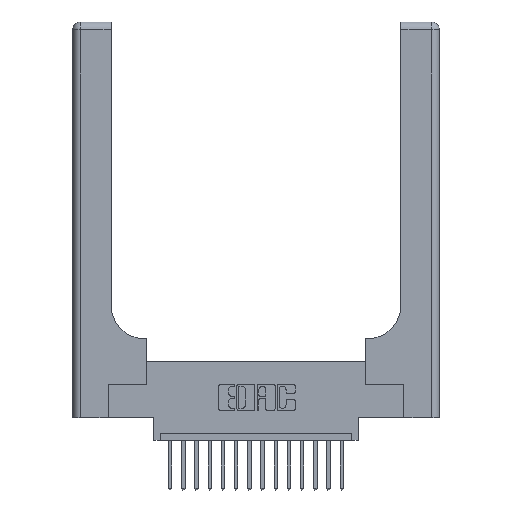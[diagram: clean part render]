
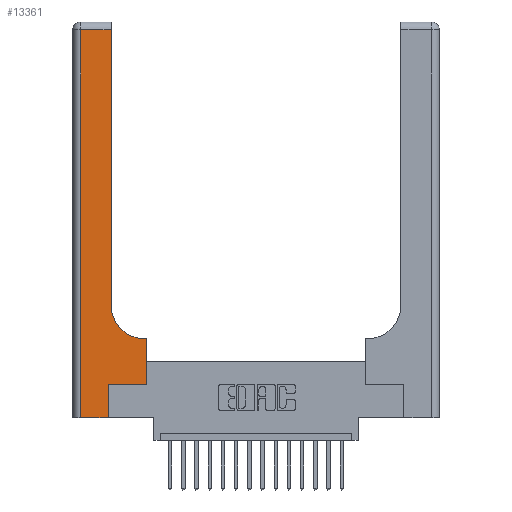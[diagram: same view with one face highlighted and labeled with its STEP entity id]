
A CAD part, top view. The second image highlights one B-rep face of the part: STEP entity #13361.
In plain terms, the highlighted planar face has unit normal (0, 0, 1).
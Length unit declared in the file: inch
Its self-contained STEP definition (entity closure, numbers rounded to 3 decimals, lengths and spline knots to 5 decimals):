
#266 = LINE ( 'NONE', #2723, #14266 ) ;
#490 = EDGE_CURVE ( 'NONE', #9068, #8698, #16690, .T. ) ;
#551 = DIRECTION ( 'NONE',  ( 1., 0., 0. ) ) ;
#700 = DIRECTION ( 'NONE',  ( 0., 0., -1. ) ) ;
#827 = ORIENTED_EDGE ( 'NONE', *, *, #14603, .T. ) ;
#1605 = DIRECTION ( 'NONE',  ( 1., 0., 0. ) ) ;
#2723 = CARTESIAN_POINT ( 'NONE',  ( 0.269, 0., 0.37 ) ) ;
#2994 = CARTESIAN_POINT ( 'NONE',  ( 0.5585, 0.6, 0.37 ) ) ;
#3148 = CARTESIAN_POINT ( 'NONE',  ( 0., 0., 0.37 ) ) ;
#3164 = CIRCLE ( 'NONE', #11990, 0.25 ) ;
#3345 = DIRECTION ( 'NONE',  ( 0., 1., 0. ) ) ;
#3385 = DIRECTION ( 'NONE',  ( 0., -1., 0. ) ) ;
#3402 = CARTESIAN_POINT ( 'NONE',  ( 0.06, 0., 0.37 ) ) ;
#3725 = CARTESIAN_POINT ( 'NONE',  ( 0.5415, 0.85, 0.37 ) ) ;
#3919 = VECTOR ( 'NONE', #551, 39.37008 ) ;
#4264 = VERTEX_POINT ( 'NONE', #17089 ) ;
#4877 = ORIENTED_EDGE ( 'NONE', *, *, #490, .T. ) ;
#5398 = VERTEX_POINT ( 'NONE', #16223 ) ;
#5767 = ORIENTED_EDGE ( 'NONE', *, *, #15978, .T. ) ;
#5943 = DIRECTION ( 'NONE',  ( 0., 1., 0. ) ) ;
#6298 = EDGE_CURVE ( 'NONE', #7502, #5398, #13728, .T. ) ;
#6806 = PLANE ( 'NONE',  #19457 ) ;
#6959 = EDGE_LOOP ( 'NONE', ( #5767, #7128, #11866, #4877, #14327, #12445, #11092, #18202, #827 ) ) ;
#7128 = ORIENTED_EDGE ( 'NONE', *, *, #6298, .T. ) ;
#7502 = VERTEX_POINT ( 'NONE', #13542 ) ;
#7515 = LINE ( 'NONE', #14103, #3919 ) ;
#8093 = DIRECTION ( 'NONE',  ( -1., 0., 0. ) ) ;
#8137 = LINE ( 'NONE', #14679, #17171 ) ;
#8184 = EDGE_CURVE ( 'NONE', #5398, #9068, #15811, .T. ) ;
#8450 = CARTESIAN_POINT ( 'NONE',  ( 0.5415, 0.6, 0.37 ) ) ;
#8490 = EDGE_CURVE ( 'NONE', #4264, #14264, #7515, .T. ) ;
#8571 = CARTESIAN_POINT ( 'NONE',  ( 0.2915, 0.85, 0.37 ) ) ;
#8698 = VERTEX_POINT ( 'NONE', #18429 ) ;
#8724 = CARTESIAN_POINT ( 'NONE',  ( 0.5585, 0.25, 0.37 ) ) ;
#9068 = VERTEX_POINT ( 'NONE', #3402 ) ;
#9424 = EDGE_CURVE ( 'NONE', #14264, #17366, #17789, .T. ) ;
#9853 = CARTESIAN_POINT ( 'NONE',  ( 0., 3., 0.37 ) ) ;
#11092 = ORIENTED_EDGE ( 'NONE', *, *, #9424, .T. ) ;
#11214 = VERTEX_POINT ( 'NONE', #8450 ) ;
#11866 = ORIENTED_EDGE ( 'NONE', *, *, #8184, .T. ) ;
#11990 = AXIS2_PLACEMENT_3D ( 'NONE', #3725, #700, #14583 ) ;
#12050 = CARTESIAN_POINT ( 'NONE',  ( 0.06, 3., 0.37 ) ) ;
#12445 = ORIENTED_EDGE ( 'NONE', *, *, #8490, .T. ) ;
#12749 = DIRECTION ( 'NONE',  ( 0., 0., -1. ) ) ;
#12912 = DIRECTION ( 'NONE',  ( 0., 1., 0. ) ) ;
#13052 = DIRECTION ( 'NONE',  ( -1., 0., 0. ) ) ;
#13361 = ADVANCED_FACE ( 'NONE', ( #14091 ), #6806, .F. ) ;
#13542 = CARTESIAN_POINT ( 'NONE',  ( 0.2915, 2.94, 0.37 ) ) ;
#13728 = LINE ( 'NONE', #18077, #16349 ) ;
#14091 = FACE_OUTER_BOUND ( 'NONE', #6959, .T. ) ;
#14103 = CARTESIAN_POINT ( 'NONE',  ( 0.269, 0.25, 0.37 ) ) ;
#14264 = VERTEX_POINT ( 'NONE', #8724 ) ;
#14266 = VECTOR ( 'NONE', #5943, 39.37008 ) ;
#14327 = ORIENTED_EDGE ( 'NONE', *, *, #14439, .T. ) ;
#14363 = VECTOR ( 'NONE', #3385, 39.37008 ) ;
#14439 = EDGE_CURVE ( 'NONE', #8698, #4264, #266, .T. ) ;
#14583 = DIRECTION ( 'NONE',  ( 1., 0., 0. ) ) ;
#14603 = EDGE_CURVE ( 'NONE', #11214, #18777, #3164, .T. ) ;
#14679 = CARTESIAN_POINT ( 'NONE',  ( 0.2915, 0.6, 0.37 ) ) ;
#15811 = LINE ( 'NONE', #12050, #14363 ) ;
#15978 = EDGE_CURVE ( 'NONE', #18777, #7502, #16131, .T. ) ;
#16062 = EDGE_CURVE ( 'NONE', #17366, #11214, #8137, .T. ) ;
#16131 = LINE ( 'NONE', #17487, #18749 ) ;
#16223 = CARTESIAN_POINT ( 'NONE',  ( 0.06, 2.94, 0.37 ) ) ;
#16349 = VECTOR ( 'NONE', #16911, 39.37008 ) ;
#16690 = LINE ( 'NONE', #3148, #18103 ) ;
#16911 = DIRECTION ( 'NONE',  ( -1., 0., 0. ) ) ;
#17089 = CARTESIAN_POINT ( 'NONE',  ( 0.269, 0.25, 0.37 ) ) ;
#17171 = VECTOR ( 'NONE', #13052, 39.37008 ) ;
#17366 = VERTEX_POINT ( 'NONE', #2994 ) ;
#17487 = CARTESIAN_POINT ( 'NONE',  ( 0.2915, 3., 0.37 ) ) ;
#17789 = LINE ( 'NONE', #18544, #18947 ) ;
#18077 = CARTESIAN_POINT ( 'NONE',  ( 0., 2.94, 0.37 ) ) ;
#18103 = VECTOR ( 'NONE', #1605, 39.37008 ) ;
#18202 = ORIENTED_EDGE ( 'NONE', *, *, #16062, .T. ) ;
#18429 = CARTESIAN_POINT ( 'NONE',  ( 0.269, 0., 0.37 ) ) ;
#18544 = CARTESIAN_POINT ( 'NONE',  ( 0.5585, 0.25, 0.37 ) ) ;
#18749 = VECTOR ( 'NONE', #12912, 39.37008 ) ;
#18777 = VERTEX_POINT ( 'NONE', #8571 ) ;
#18947 = VECTOR ( 'NONE', #3345, 39.37008 ) ;
#19457 = AXIS2_PLACEMENT_3D ( 'NONE', #9853, #12749, #8093 ) ;
